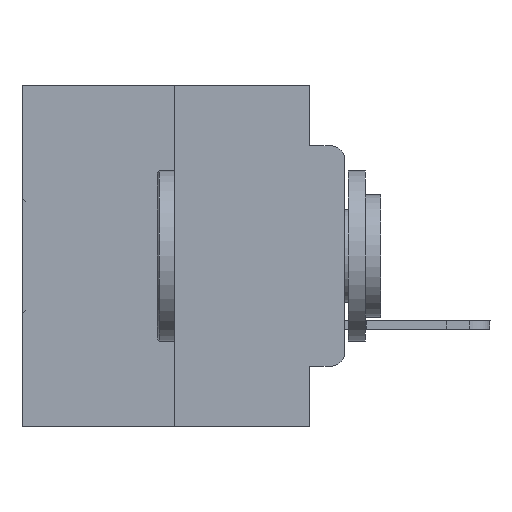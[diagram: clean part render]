
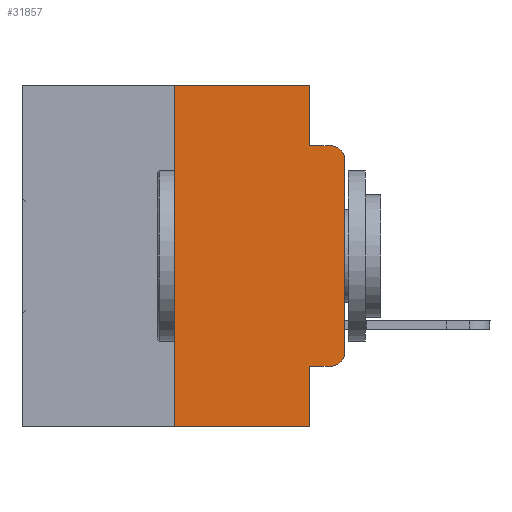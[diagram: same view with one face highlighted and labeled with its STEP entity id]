
A CAD part, left-side view. The second image highlights one B-rep face of the part: STEP entity #31857.
In plain terms, the highlighted planar face has unit normal (-1, 0, 0).
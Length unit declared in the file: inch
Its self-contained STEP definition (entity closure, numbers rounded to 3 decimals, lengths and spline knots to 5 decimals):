
#942 = CARTESIAN_POINT ( 'NONE',  ( 0., 0.02, -0.3915 ) ) ;
#1042 = EDGE_CURVE ( 'NONE', #24293, #24100, #9592, .T. ) ;
#1719 = EDGE_CURVE ( 'NONE', #8625, #19167, #22315, .T. ) ;
#1785 = EDGE_CURVE ( 'NONE', #29672, #24100, #9144, .T. ) ;
#2413 = VECTOR ( 'NONE', #26954, 39.37008 ) ;
#2484 = ORIENTED_EDGE ( 'NONE', *, *, #11683, .F. ) ;
#3315 = CARTESIAN_POINT ( 'NONE',  ( 0., 0., -0.1085 ) ) ;
#3370 = CARTESIAN_POINT ( 'NONE',  ( 0., 0.051, -0.4115 ) ) ;
#3672 = ORIENTED_EDGE ( 'NONE', *, *, #1719, .T. ) ;
#3911 = CARTESIAN_POINT ( 'NONE',  ( 0., 0.473, -0.5 ) ) ;
#4129 = EDGE_CURVE ( 'NONE', #8625, #24980, #15600, .T. ) ;
#4822 = ORIENTED_EDGE ( 'NONE', *, *, #19482, .F. ) ;
#4856 = CARTESIAN_POINT ( 'NONE',  ( 0., 0.02, -0.0885 ) ) ;
#4950 = CARTESIAN_POINT ( 'NONE',  ( 0., 0.473, 0. ) ) ;
#4953 = VECTOR ( 'NONE', #18025, 39.37008 ) ;
#5365 = DIRECTION ( 'NONE',  ( 0., 0., 1. ) ) ;
#5680 = CARTESIAN_POINT ( 'NONE',  ( 0., 0.051, -0.4115 ) ) ;
#6738 = VECTOR ( 'NONE', #5365, 39.37008 ) ;
#6809 = CARTESIAN_POINT ( 'NONE',  ( 0., 0.051, -0.0885 ) ) ;
#6916 = VECTOR ( 'NONE', #18050, 39.37008 ) ;
#7420 = VERTEX_POINT ( 'NONE', #12908 ) ;
#7601 = ORIENTED_EDGE ( 'NONE', *, *, #1785, .F. ) ;
#8164 = DIRECTION ( 'NONE',  ( 0., 0., -1. ) ) ;
#8365 = VECTOR ( 'NONE', #19538, 39.37008 ) ;
#8396 = VECTOR ( 'NONE', #28604, 39.37008 ) ;
#8625 = VERTEX_POINT ( 'NONE', #24552 ) ;
#9116 = EDGE_CURVE ( 'NONE', #15280, #19167, #28953, .T. ) ;
#9144 = LINE ( 'NONE', #6809, #8365 ) ;
#9359 = ORIENTED_EDGE ( 'NONE', *, *, #9878, .T. ) ;
#9592 = CIRCLE ( 'NONE', #22641, 0.02 ) ;
#9878 = EDGE_CURVE ( 'NONE', #7420, #11950, #16907, .T. ) ;
#10524 = DIRECTION ( 'NONE',  ( -1., 0., 0. ) ) ;
#11606 = DIRECTION ( 'NONE',  ( 0., 0., -1. ) ) ;
#11683 = EDGE_CURVE ( 'NONE', #31604, #29672, #13910, .T. ) ;
#11950 = VERTEX_POINT ( 'NONE', #21697 ) ;
#12197 = CARTESIAN_POINT ( 'NONE',  ( 0., 0.051, 0. ) ) ;
#12338 = AXIS2_PLACEMENT_3D ( 'NONE', #942, #10524, #8164 ) ;
#12908 = CARTESIAN_POINT ( 'NONE',  ( 0., 0.02, -0.4115 ) ) ;
#13910 = LINE ( 'NONE', #28192, #20851 ) ;
#13940 = FACE_OUTER_BOUND ( 'NONE', #20735, .T. ) ;
#15280 = VERTEX_POINT ( 'NONE', #5680 ) ;
#15600 = LINE ( 'NONE', #27268, #6738 ) ;
#16015 = PLANE ( 'NONE',  #23984 ) ;
#16337 = DIRECTION ( 'NONE',  ( 1., 0., 0. ) ) ;
#16907 = CIRCLE ( 'NONE', #12338, 0.02 ) ;
#17886 = ORIENTED_EDGE ( 'NONE', *, *, #4129, .F. ) ;
#18025 = DIRECTION ( 'NONE',  ( 0., -1., 0. ) ) ;
#18050 = DIRECTION ( 'NONE',  ( 0., 0., 1. ) ) ;
#18497 = CARTESIAN_POINT ( 'NONE',  ( 0., 0.473, 0. ) ) ;
#18625 = ORIENTED_EDGE ( 'NONE', *, *, #22226, .T. ) ;
#19167 = VERTEX_POINT ( 'NONE', #30815 ) ;
#19482 = EDGE_CURVE ( 'NONE', #24980, #31604, #22105, .T. ) ;
#19538 = DIRECTION ( 'NONE',  ( 0., -1., 0. ) ) ;
#20411 = DIRECTION ( 'NONE',  ( 0., 0., -1. ) ) ;
#20422 = CARTESIAN_POINT ( 'NONE',  ( 0., 0.25, 0. ) ) ;
#20456 = VECTOR ( 'NONE', #21840, 39.37008 ) ;
#20735 = EDGE_LOOP ( 'NONE', ( #21517, #22694, #7601, #2484, #4822, #17886, #3672, #25501, #18625, #9359 ) ) ;
#20851 = VECTOR ( 'NONE', #20411, 39.37008 ) ;
#21517 = ORIENTED_EDGE ( 'NONE', *, *, #21693, .T. ) ;
#21693 = EDGE_CURVE ( 'NONE', #11950, #24293, #28171, .T. ) ;
#21697 = CARTESIAN_POINT ( 'NONE',  ( 0., 0., -0.3915 ) ) ;
#21840 = DIRECTION ( 'NONE',  ( 0., 0., -1. ) ) ;
#22105 = LINE ( 'NONE', #4950, #2413 ) ;
#22226 = EDGE_CURVE ( 'NONE', #15280, #7420, #31938, .T. ) ;
#22315 = LINE ( 'NONE', #3911, #8396 ) ;
#22641 = AXIS2_PLACEMENT_3D ( 'NONE', #26757, #26437, #11606 ) ;
#22694 = ORIENTED_EDGE ( 'NONE', *, *, #1042, .T. ) ;
#23984 = AXIS2_PLACEMENT_3D ( 'NONE', #18497, #16337, #28547 ) ;
#24100 = VERTEX_POINT ( 'NONE', #4856 ) ;
#24293 = VERTEX_POINT ( 'NONE', #3315 ) ;
#24552 = CARTESIAN_POINT ( 'NONE',  ( 0., 0.25, -0.5 ) ) ;
#24980 = VERTEX_POINT ( 'NONE', #20422 ) ;
#25501 = ORIENTED_EDGE ( 'NONE', *, *, #9116, .F. ) ;
#26437 = DIRECTION ( 'NONE',  ( -1., 0., 0. ) ) ;
#26757 = CARTESIAN_POINT ( 'NONE',  ( 0., 0.02, -0.1085 ) ) ;
#26954 = DIRECTION ( 'NONE',  ( 0., -1., 0. ) ) ;
#27268 = CARTESIAN_POINT ( 'NONE',  ( 0., 0.25, 0. ) ) ;
#27313 = CARTESIAN_POINT ( 'NONE',  ( 0., 0.051, -0.0885 ) ) ;
#27592 = CARTESIAN_POINT ( 'NONE',  ( 0., 0.051, 0. ) ) ;
#28171 = LINE ( 'NONE', #28328, #6916 ) ;
#28192 = CARTESIAN_POINT ( 'NONE',  ( 0., 0.051, 0. ) ) ;
#28328 = CARTESIAN_POINT ( 'NONE',  ( 0., 0., 0. ) ) ;
#28547 = DIRECTION ( 'NONE',  ( 0., 0., -1. ) ) ;
#28604 = DIRECTION ( 'NONE',  ( 0., -1., 0. ) ) ;
#28953 = LINE ( 'NONE', #12197, #20456 ) ;
#29672 = VERTEX_POINT ( 'NONE', #27313 ) ;
#30815 = CARTESIAN_POINT ( 'NONE',  ( 0., 0.051, -0.5 ) ) ;
#31604 = VERTEX_POINT ( 'NONE', #27592 ) ;
#31857 = ADVANCED_FACE ( 'NONE', ( #13940 ), #16015, .F. ) ;
#31938 = LINE ( 'NONE', #3370, #4953 ) ;
